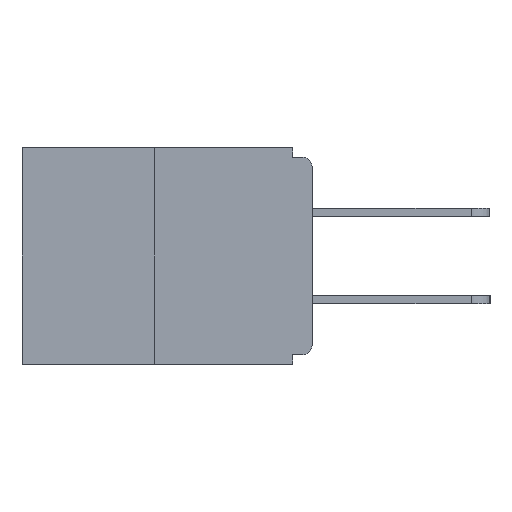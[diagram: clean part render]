
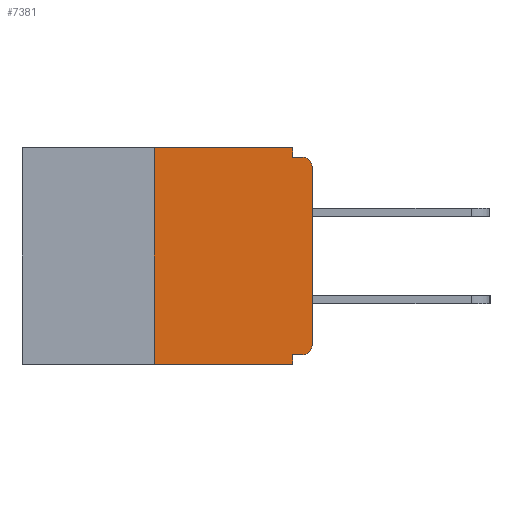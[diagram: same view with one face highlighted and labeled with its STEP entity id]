
A CAD part, left-side view. The second image highlights one B-rep face of the part: STEP entity #7381.
In plain terms, the highlighted planar face has unit normal (-1, 0, 0).
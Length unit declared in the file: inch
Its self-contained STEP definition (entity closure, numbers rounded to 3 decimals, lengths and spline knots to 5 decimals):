
#37 = CARTESIAN_POINT ( 'NONE',  ( 0., 0.031, 0. ) ) ;
#110 = DIRECTION ( 'NONE',  ( 0., 0., -1. ) ) ;
#235 = EDGE_CURVE ( 'NONE', #2941, #10669, #10552, .T. ) ;
#496 = FACE_OUTER_BOUND ( 'NONE', #2242, .T. ) ;
#692 = AXIS2_PLACEMENT_3D ( 'NONE', #1093, #2635, #12821 ) ;
#941 = VERTEX_POINT ( 'NONE', #9573 ) ;
#1093 = CARTESIAN_POINT ( 'NONE',  ( 0., 0.015, -0.313 ) ) ;
#2138 = PLANE ( 'NONE',  #3633 ) ;
#2235 = CIRCLE ( 'NONE', #692, 0.015 ) ;
#2242 = EDGE_LOOP ( 'NONE', ( #3541, #8170, #14328, #10872, #5756, #13051, #15952, #5689, #8418, #3639 ) ) ;
#2446 = CARTESIAN_POINT ( 'NONE',  ( 0., 0., -0.015 ) ) ;
#2504 = CARTESIAN_POINT ( 'NONE',  ( 0., 0.031, -0.328 ) ) ;
#2635 = DIRECTION ( 'NONE',  ( -1., 0., 0. ) ) ;
#2941 = VERTEX_POINT ( 'NONE', #4858 ) ;
#2945 = EDGE_CURVE ( 'NONE', #18737, #5092, #6123, .T. ) ;
#2977 = VECTOR ( 'NONE', #9530, 39.37008 ) ;
#3066 = CARTESIAN_POINT ( 'NONE',  ( 0., 0.46, -0.343 ) ) ;
#3144 = DIRECTION ( 'NONE',  ( 0., 1., 0. ) ) ;
#3488 = CARTESIAN_POINT ( 'NONE',  ( 0., 0.46, 0. ) ) ;
#3541 = ORIENTED_EDGE ( 'NONE', *, *, #2945, .F. ) ;
#3633 = AXIS2_PLACEMENT_3D ( 'NONE', #3488, #13836, #10979 ) ;
#3639 = ORIENTED_EDGE ( 'NONE', *, *, #15796, .F. ) ;
#3777 = DIRECTION ( 'NONE',  ( 0., -1., 0. ) ) ;
#4034 = LINE ( 'NONE', #11428, #2977 ) ;
#4747 = VERTEX_POINT ( 'NONE', #11694 ) ;
#4819 = VERTEX_POINT ( 'NONE', #13674 ) ;
#4858 = CARTESIAN_POINT ( 'NONE',  ( 0., 0., -0.03 ) ) ;
#5092 = VERTEX_POINT ( 'NONE', #37 ) ;
#5125 = LINE ( 'NONE', #2446, #8021 ) ;
#5606 = CARTESIAN_POINT ( 'NONE',  ( 0., 0.031, 0. ) ) ;
#5689 = ORIENTED_EDGE ( 'NONE', *, *, #235, .T. ) ;
#5756 = ORIENTED_EDGE ( 'NONE', *, *, #9079, .F. ) ;
#5774 = DIRECTION ( 'NONE',  ( 0., 0., -1. ) ) ;
#6123 = LINE ( 'NONE', #17839, #7206 ) ;
#6220 = CARTESIAN_POINT ( 'NONE',  ( 0., 0.015, -0.015 ) ) ;
#6922 = CARTESIAN_POINT ( 'NONE',  ( 0., 0., 0. ) ) ;
#7005 = VECTOR ( 'NONE', #17092, 39.37008 ) ;
#7206 = VECTOR ( 'NONE', #7469, 39.37008 ) ;
#7294 = VERTEX_POINT ( 'NONE', #15713 ) ;
#7326 = VECTOR ( 'NONE', #10035, 39.37008 ) ;
#7381 = ADVANCED_FACE ( 'NONE', ( #496 ), #2138, .F. ) ;
#7469 = DIRECTION ( 'NONE',  ( 0., -1., 0. ) ) ;
#8021 = VECTOR ( 'NONE', #3777, 39.37008 ) ;
#8170 = ORIENTED_EDGE ( 'NONE', *, *, #8225, .F. ) ;
#8190 = VERTEX_POINT ( 'NONE', #2504 ) ;
#8225 = EDGE_CURVE ( 'NONE', #7294, #18737, #4034, .T. ) ;
#8418 = ORIENTED_EDGE ( 'NONE', *, *, #12732, .F. ) ;
#8818 = VECTOR ( 'NONE', #3144, 39.37008 ) ;
#9079 = EDGE_CURVE ( 'NONE', #12754, #8190, #9388, .T. ) ;
#9151 = VECTOR ( 'NONE', #17485, 39.37008 ) ;
#9388 = LINE ( 'NONE', #16304, #8818 ) ;
#9530 = DIRECTION ( 'NONE',  ( 0., 0., 1. ) ) ;
#9573 = CARTESIAN_POINT ( 'NONE',  ( 0., 0.031, -0.343 ) ) ;
#9655 = CARTESIAN_POINT ( 'NONE',  ( 0., 0.25, 0. ) ) ;
#10035 = DIRECTION ( 'NONE',  ( 0., 0., -1. ) ) ;
#10083 = EDGE_CURVE ( 'NONE', #7294, #941, #12951, .T. ) ;
#10552 = CIRCLE ( 'NONE', #18525, 0.015 ) ;
#10669 = VERTEX_POINT ( 'NONE', #6220 ) ;
#10872 = ORIENTED_EDGE ( 'NONE', *, *, #14671, .F. ) ;
#10979 = DIRECTION ( 'NONE',  ( 0., 0., -1. ) ) ;
#11135 = LINE ( 'NONE', #6922, #7005 ) ;
#11428 = CARTESIAN_POINT ( 'NONE',  ( 0., 0.25, 0. ) ) ;
#11694 = CARTESIAN_POINT ( 'NONE',  ( 0., 0.031, -0.015 ) ) ;
#11778 = EDGE_CURVE ( 'NONE', #4819, #2941, #11135, .T. ) ;
#11818 = CARTESIAN_POINT ( 'NONE',  ( 0., 0.015, -0.03 ) ) ;
#12242 = CARTESIAN_POINT ( 'NONE',  ( 0., 0.015, -0.328 ) ) ;
#12732 = EDGE_CURVE ( 'NONE', #4747, #10669, #5125, .T. ) ;
#12754 = VERTEX_POINT ( 'NONE', #12242 ) ;
#12821 = DIRECTION ( 'NONE',  ( 0., 0., -1. ) ) ;
#12951 = LINE ( 'NONE', #3066, #9151 ) ;
#13051 = ORIENTED_EDGE ( 'NONE', *, *, #14111, .T. ) ;
#13367 = LINE ( 'NONE', #16445, #17610 ) ;
#13674 = CARTESIAN_POINT ( 'NONE',  ( 0., 0., -0.313 ) ) ;
#13836 = DIRECTION ( 'NONE',  ( 1., 0., 0. ) ) ;
#14111 = EDGE_CURVE ( 'NONE', #12754, #4819, #2235, .T. ) ;
#14328 = ORIENTED_EDGE ( 'NONE', *, *, #10083, .T. ) ;
#14671 = EDGE_CURVE ( 'NONE', #8190, #941, #13367, .T. ) ;
#15713 = CARTESIAN_POINT ( 'NONE',  ( 0., 0.25, -0.343 ) ) ;
#15796 = EDGE_CURVE ( 'NONE', #5092, #4747, #18780, .T. ) ;
#15952 = ORIENTED_EDGE ( 'NONE', *, *, #11778, .T. ) ;
#16304 = CARTESIAN_POINT ( 'NONE',  ( 0., 0., -0.328 ) ) ;
#16445 = CARTESIAN_POINT ( 'NONE',  ( 0., 0.031, -0.343 ) ) ;
#17092 = DIRECTION ( 'NONE',  ( 0., 0., 1. ) ) ;
#17485 = DIRECTION ( 'NONE',  ( 0., -1., 0. ) ) ;
#17610 = VECTOR ( 'NONE', #110, 39.37008 ) ;
#17839 = CARTESIAN_POINT ( 'NONE',  ( 0., 0.46, 0. ) ) ;
#18525 = AXIS2_PLACEMENT_3D ( 'NONE', #11818, #18853, #5774 ) ;
#18737 = VERTEX_POINT ( 'NONE', #9655 ) ;
#18780 = LINE ( 'NONE', #5606, #7326 ) ;
#18853 = DIRECTION ( 'NONE',  ( -1., 0., 0. ) ) ;
